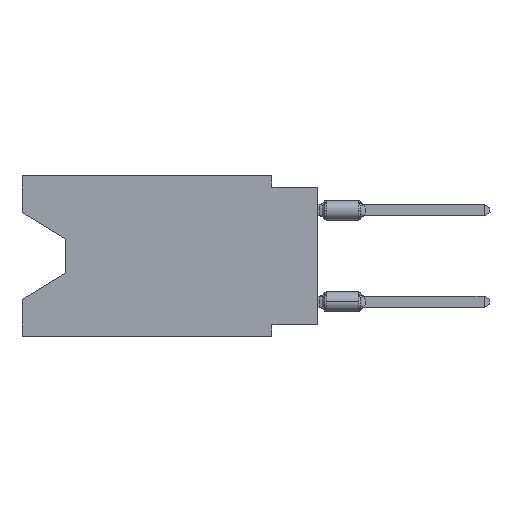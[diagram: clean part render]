
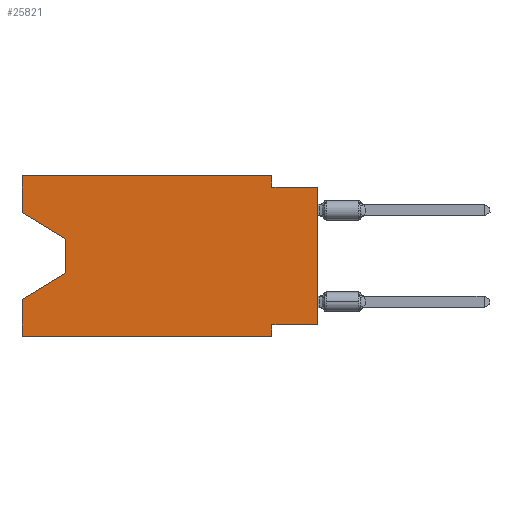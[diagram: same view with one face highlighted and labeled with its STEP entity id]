
A CAD part, left-side view. The second image highlights one B-rep face of the part: STEP entity #25821.
In plain terms, the highlighted planar face has unit normal (-1, 0, 0).
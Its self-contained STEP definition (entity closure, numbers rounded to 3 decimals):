
#170 = EDGE_CURVE ( 'NONE', #23367, #9634, #7671, .T. ) ;
#176 = DIRECTION ( 'NONE',  ( 0., 0., 1. ) ) ;
#339 = CARTESIAN_POINT ( 'NONE',  ( 0., 0., -8.255 ) ) ;
#959 = VERTEX_POINT ( 'NONE', #339 ) ;
#1159 = ORIENTED_EDGE ( 'NONE', *, *, #9071, .F. ) ;
#1733 = LINE ( 'NONE', #15050, #9843 ) ;
#1741 = CARTESIAN_POINT ( 'NONE',  ( 0., 16.383, 0. ) ) ;
#1833 = CARTESIAN_POINT ( 'NONE',  ( 0., 16.383, -2.038 ) ) ;
#2004 = PLANE ( 'NONE',  #10515 ) ;
#2257 = CARTESIAN_POINT ( 'NONE',  ( 0., 13.97, -3.505 ) ) ;
#2495 = VECTOR ( 'NONE', #26113, 1000. ) ;
#2844 = VERTEX_POINT ( 'NONE', #22492 ) ;
#3321 = EDGE_LOOP ( 'NONE', ( #11907, #20000, #7181, #9776, #18876, #6255, #17150, #16431, #1159, #9383, #9002, #11450 ) ) ;
#3520 = DIRECTION ( 'NONE',  ( 0., 0., -1. ) ) ;
#4308 = CARTESIAN_POINT ( 'NONE',  ( 0., 16.383, -8.89 ) ) ;
#5272 = EDGE_CURVE ( 'NONE', #959, #24777, #9207, .T. ) ;
#5385 = VERTEX_POINT ( 'NONE', #10399 ) ;
#5698 = DIRECTION ( 'NONE',  ( 0., 0., -1. ) ) ;
#5814 = VECTOR ( 'NONE', #14382, 1000. ) ;
#5910 = VECTOR ( 'NONE', #7599, 1000. ) ;
#5919 = CARTESIAN_POINT ( 'NONE',  ( 0., 16.383, 0. ) ) ;
#6255 = ORIENTED_EDGE ( 'NONE', *, *, #10536, .F. ) ;
#6351 = DIRECTION ( 'NONE',  ( 0., 0., 1. ) ) ;
#6354 = VECTOR ( 'NONE', #27263, 1000. ) ;
#6662 = LINE ( 'NONE', #4308, #14107 ) ;
#7181 = ORIENTED_EDGE ( 'NONE', *, *, #25239, .T. ) ;
#7532 = VERTEX_POINT ( 'NONE', #8443 ) ;
#7599 = DIRECTION ( 'NONE',  ( 0., -1., 0. ) ) ;
#7630 = VECTOR ( 'NONE', #24218, 1000. ) ;
#7671 = LINE ( 'NONE', #14214, #22949 ) ;
#7962 = LINE ( 'NONE', #11193, #14537 ) ;
#8254 = LINE ( 'NONE', #1741, #5814 ) ;
#8443 = CARTESIAN_POINT ( 'NONE',  ( 0., 2.54, -0.635 ) ) ;
#9002 = ORIENTED_EDGE ( 'NONE', *, *, #15829, .F. ) ;
#9071 = EDGE_CURVE ( 'NONE', #7532, #5385, #27019, .T. ) ;
#9207 = LINE ( 'NONE', #17674, #2495 ) ;
#9383 = ORIENTED_EDGE ( 'NONE', *, *, #23215, .F. ) ;
#9594 = EDGE_CURVE ( 'NONE', #959, #5385, #1733, .T. ) ;
#9634 = VERTEX_POINT ( 'NONE', #2257 ) ;
#9776 = ORIENTED_EDGE ( 'NONE', *, *, #17334, .F. ) ;
#9843 = VECTOR ( 'NONE', #176, 1000. ) ;
#10357 = LINE ( 'NONE', #17013, #6354 ) ;
#10395 = CARTESIAN_POINT ( 'NONE',  ( 0., 13.97, -3.505 ) ) ;
#10399 = CARTESIAN_POINT ( 'NONE',  ( 0., 0., -0.635 ) ) ;
#10515 = AXIS2_PLACEMENT_3D ( 'NONE', #5919, #27011, #16609 ) ;
#10536 = EDGE_CURVE ( 'NONE', #24777, #23285, #21860, .T. ) ;
#10805 = VERTEX_POINT ( 'NONE', #14911 ) ;
#11193 = CARTESIAN_POINT ( 'NONE',  ( 0., 2.54, 0. ) ) ;
#11450 = ORIENTED_EDGE ( 'NONE', *, *, #12176, .F. ) ;
#11726 = CARTESIAN_POINT ( 'NONE',  ( 0., 2.54, 0. ) ) ;
#11907 = ORIENTED_EDGE ( 'NONE', *, *, #170, .T. ) ;
#12144 = CARTESIAN_POINT ( 'NONE',  ( 0., 13.97, -5.385 ) ) ;
#12176 = EDGE_CURVE ( 'NONE', #23367, #25136, #8254, .T. ) ;
#12181 = FACE_OUTER_BOUND ( 'NONE', #3321, .T. ) ;
#12404 = CARTESIAN_POINT ( 'NONE',  ( 0., 2.54, -8.89 ) ) ;
#14107 = VECTOR ( 'NONE', #21506, 1000. ) ;
#14214 = CARTESIAN_POINT ( 'NONE',  ( 0., 16.383, -2.038 ) ) ;
#14382 = DIRECTION ( 'NONE',  ( 0., 0., 1. ) ) ;
#14537 = VECTOR ( 'NONE', #3520, 1000. ) ;
#14691 = VECTOR ( 'NONE', #5698, 1000. ) ;
#14753 = CARTESIAN_POINT ( 'NONE',  ( 0., 16.383, 0. ) ) ;
#14911 = CARTESIAN_POINT ( 'NONE',  ( 0., 16.383, -6.852 ) ) ;
#15050 = CARTESIAN_POINT ( 'NONE',  ( 0., 0., 0. ) ) ;
#15760 = CARTESIAN_POINT ( 'NONE',  ( 0., 2.54, -8.89 ) ) ;
#15829 = EDGE_CURVE ( 'NONE', #25136, #26024, #10357, .T. ) ;
#15880 = DIRECTION ( 'NONE',  ( 0., -0.855, -0.519 ) ) ;
#15960 = CARTESIAN_POINT ( 'NONE',  ( 0., 13.97, -5.385 ) ) ;
#16431 = ORIENTED_EDGE ( 'NONE', *, *, #9594, .T. ) ;
#16609 = DIRECTION ( 'NONE',  ( 0., 0., -1. ) ) ;
#16729 = EDGE_CURVE ( 'NONE', #2844, #23285, #6662, .T. ) ;
#17013 = CARTESIAN_POINT ( 'NONE',  ( 0., 16.383, 0. ) ) ;
#17068 = EDGE_CURVE ( 'NONE', #9634, #21241, #26914, .T. ) ;
#17150 = ORIENTED_EDGE ( 'NONE', *, *, #5272, .F. ) ;
#17334 = EDGE_CURVE ( 'NONE', #2844, #10805, #19011, .T. ) ;
#17674 = CARTESIAN_POINT ( 'NONE',  ( 0., 0., -8.255 ) ) ;
#17902 = LINE ( 'NONE', #15960, #18504 ) ;
#18504 = VECTOR ( 'NONE', #24544, 1000. ) ;
#18876 = ORIENTED_EDGE ( 'NONE', *, *, #16729, .T. ) ;
#19011 = LINE ( 'NONE', #22122, #20440 ) ;
#19098 = CARTESIAN_POINT ( 'NONE',  ( 0., 2.54, -8.255 ) ) ;
#20000 = ORIENTED_EDGE ( 'NONE', *, *, #17068, .T. ) ;
#20440 = VECTOR ( 'NONE', #6351, 1000. ) ;
#20512 = CARTESIAN_POINT ( 'NONE',  ( 0., 0., -0.635 ) ) ;
#21241 = VERTEX_POINT ( 'NONE', #12144 ) ;
#21506 = DIRECTION ( 'NONE',  ( 0., -1., 0. ) ) ;
#21860 = LINE ( 'NONE', #15760, #7630 ) ;
#22122 = CARTESIAN_POINT ( 'NONE',  ( 0., 16.383, 0. ) ) ;
#22492 = CARTESIAN_POINT ( 'NONE',  ( 0., 16.383, -8.89 ) ) ;
#22949 = VECTOR ( 'NONE', #15880, 1000. ) ;
#23215 = EDGE_CURVE ( 'NONE', #26024, #7532, #7962, .T. ) ;
#23285 = VERTEX_POINT ( 'NONE', #12404 ) ;
#23367 = VERTEX_POINT ( 'NONE', #1833 ) ;
#24218 = DIRECTION ( 'NONE',  ( 0., 0., -1. ) ) ;
#24544 = DIRECTION ( 'NONE',  ( 0., 0.855, -0.519 ) ) ;
#24777 = VERTEX_POINT ( 'NONE', #19098 ) ;
#25136 = VERTEX_POINT ( 'NONE', #14753 ) ;
#25239 = EDGE_CURVE ( 'NONE', #21241, #10805, #17902, .T. ) ;
#25821 = ADVANCED_FACE ( 'NONE', ( #12181 ), #2004, .F. ) ;
#26024 = VERTEX_POINT ( 'NONE', #11726 ) ;
#26113 = DIRECTION ( 'NONE',  ( 0., 1., 0. ) ) ;
#26914 = LINE ( 'NONE', #10395, #14691 ) ;
#27011 = DIRECTION ( 'NONE',  ( 1., 0., 0. ) ) ;
#27019 = LINE ( 'NONE', #20512, #5910 ) ;
#27263 = DIRECTION ( 'NONE',  ( 0., -1., 0. ) ) ;
